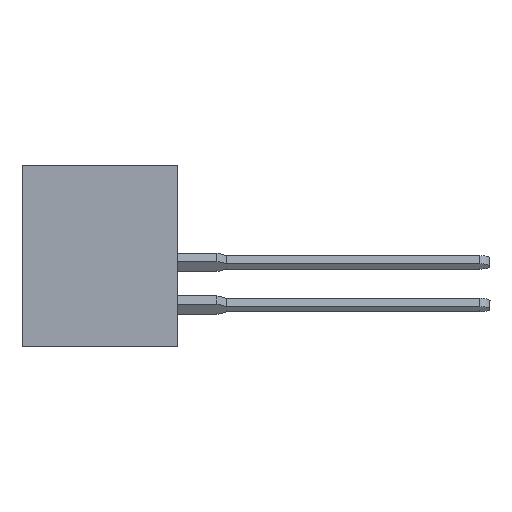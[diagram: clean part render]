
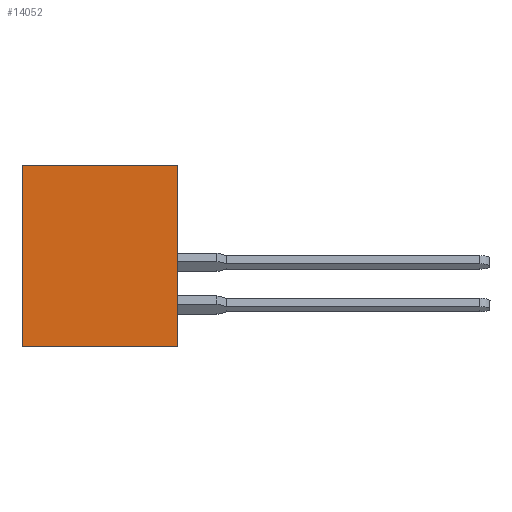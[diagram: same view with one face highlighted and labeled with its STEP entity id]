
A CAD part, left-side view. The second image highlights one B-rep face of the part: STEP entity #14052.
In plain terms, the highlighted planar face has unit normal (-1, 0, 0).
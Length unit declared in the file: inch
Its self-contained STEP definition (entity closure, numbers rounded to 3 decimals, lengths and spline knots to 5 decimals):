
#435 = VECTOR ( 'NONE', #23752, 39.37008 ) ;
#769 = DIRECTION ( 'NONE',  ( 0., -1., 0. ) ) ;
#1465 = CARTESIAN_POINT ( 'NONE',  ( 0., 0.453, 0. ) ) ;
#1961 = VERTEX_POINT ( 'NONE', #8486 ) ;
#2621 = CARTESIAN_POINT ( 'NONE',  ( 0., 0., 0. ) ) ;
#2812 = AXIS2_PLACEMENT_3D ( 'NONE', #20372, #3845, #5886 ) ;
#3278 = LINE ( 'NONE', #21225, #17676 ) ;
#3845 = DIRECTION ( 'NONE',  ( 1., 0., 0. ) ) ;
#5610 = LINE ( 'NONE', #13286, #20333 ) ;
#5886 = DIRECTION ( 'NONE',  ( 0., 0., -1. ) ) ;
#5898 = DIRECTION ( 'NONE',  ( 0., 0., 1. ) ) ;
#8096 = LINE ( 'NONE', #23664, #435 ) ;
#8486 = CARTESIAN_POINT ( 'NONE',  ( 0., 0.453, -0.531 ) ) ;
#9045 = EDGE_CURVE ( 'NONE', #9411, #17646, #5610, .T. ) ;
#9411 = VERTEX_POINT ( 'NONE', #12485 ) ;
#11034 = EDGE_LOOP ( 'NONE', ( #23875, #15244, #25798, #12672 ) ) ;
#12405 = LINE ( 'NONE', #1465, #18499 ) ;
#12485 = CARTESIAN_POINT ( 'NONE',  ( 0., 0., -0.531 ) ) ;
#12672 = ORIENTED_EDGE ( 'NONE', *, *, #18942, .T. ) ;
#13286 = CARTESIAN_POINT ( 'NONE',  ( 0., 0., 0. ) ) ;
#14052 = ADVANCED_FACE ( 'NONE', ( #24221 ), #14483, .F. ) ;
#14483 = PLANE ( 'NONE',  #2812 ) ;
#15244 = ORIENTED_EDGE ( 'NONE', *, *, #21957, .F. ) ;
#17646 = VERTEX_POINT ( 'NONE', #2621 ) ;
#17676 = VECTOR ( 'NONE', #769, 39.37008 ) ;
#18499 = VECTOR ( 'NONE', #5898, 39.37008 ) ;
#18942 = EDGE_CURVE ( 'NONE', #1961, #9411, #8096, .T. ) ;
#19233 = DIRECTION ( 'NONE',  ( 0., 0., 1. ) ) ;
#20333 = VECTOR ( 'NONE', #19233, 39.37008 ) ;
#20372 = CARTESIAN_POINT ( 'NONE',  ( 0., 0.453, 0. ) ) ;
#21225 = CARTESIAN_POINT ( 'NONE',  ( 0., 0.453, 0. ) ) ;
#21957 = EDGE_CURVE ( 'NONE', #23673, #17646, #3278, .T. ) ;
#23664 = CARTESIAN_POINT ( 'NONE',  ( 0., 0.453, -0.531 ) ) ;
#23673 = VERTEX_POINT ( 'NONE', #24889 ) ;
#23752 = DIRECTION ( 'NONE',  ( 0., -1., 0. ) ) ;
#23875 = ORIENTED_EDGE ( 'NONE', *, *, #9045, .T. ) ;
#24031 = EDGE_CURVE ( 'NONE', #1961, #23673, #12405, .T. ) ;
#24221 = FACE_OUTER_BOUND ( 'NONE', #11034, .T. ) ;
#24889 = CARTESIAN_POINT ( 'NONE',  ( 0., 0.453, 0. ) ) ;
#25798 = ORIENTED_EDGE ( 'NONE', *, *, #24031, .F. ) ;
